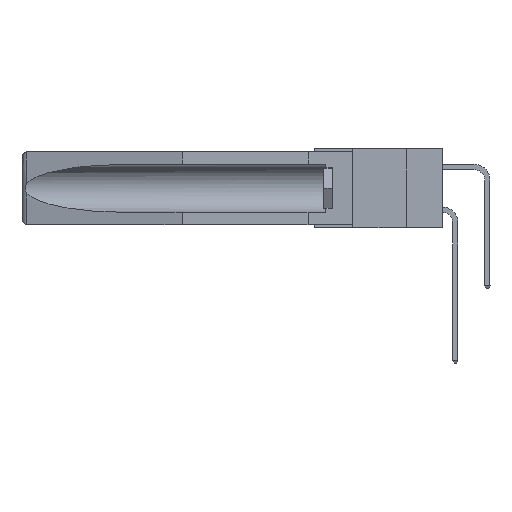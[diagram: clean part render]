
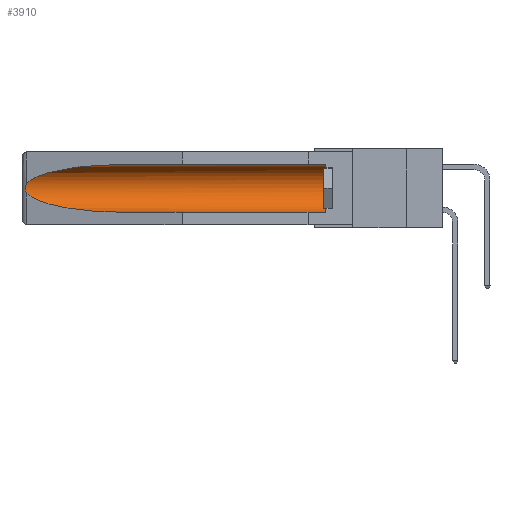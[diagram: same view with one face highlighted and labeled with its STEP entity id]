
A CAD part, left-side view. The second image highlights one B-rep face of the part: STEP entity #3910.
In plain terms, the highlighted cylindrical face has radius 2.857 mm (diameter 5.715 mm), a partial arc.
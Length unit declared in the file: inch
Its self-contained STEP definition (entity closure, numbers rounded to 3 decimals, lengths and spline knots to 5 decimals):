
#23 = CARTESIAN_POINT ( 'NONE',  ( 0.25451, 1.48313, -0.24835 ) ) ;
#266 = ORIENTED_EDGE ( 'NONE', *, *, #12073, .T. ) ;
#439 = EDGE_CURVE ( 'NONE', #23242, #6921, #13004, .T. ) ;
#444 = ORIENTED_EDGE ( 'NONE', *, *, #19345, .F. ) ;
#2038 = DIRECTION ( 'NONE',  ( 0., 0., 1. ) ) ;
#3085 = CARTESIAN_POINT ( 'NONE',  ( 0.26537, 1.52718, -0.14972 ) ) ;
#3279 = DIRECTION ( 'NONE',  ( 0., 1., 0. ) ) ;
#3375 = CARTESIAN_POINT ( 'NONE',  ( 0.26537, 1.52718, -0.19328 ) ) ;
#3388 = LINE ( 'NONE', #18462, #26644 ) ;
#3910 = ADVANCED_FACE ( 'NONE', ( #24500 ), #26945, .F. ) ;
#4541 = CARTESIAN_POINT ( 'NONE',  ( 0.155, 1.07973, -0.284 ) ) ;
#5768 = CARTESIAN_POINT ( 'NONE',  ( 0.155, 1.07973, -0.059 ) ) ;
#5815 = AXIS2_PLACEMENT_3D ( 'NONE', #20556, #8713, #2038 ) ;
#6285 = CIRCLE ( 'NONE', #5815, 0.1125 ) ;
#6734 = CARTESIAN_POINT ( 'NONE',  ( 0.26537, 1.52718, -0.14972 ) ) ;
#6921 = VERTEX_POINT ( 'NONE', #12765 ) ;
#7908 = ORIENTED_EDGE ( 'NONE', *, *, #19481, .T. ) ;
#7948 = VECTOR ( 'NONE', #3279, 39.37008 ) ;
#8572 = EDGE_LOOP ( 'NONE', ( #20658, #13255, #21803, #444, #266, #7908 ) ) ;
#8713 = DIRECTION ( 'NONE',  ( 0., -1., 0. ) ) ;
#8880 = CARTESIAN_POINT ( 'NONE',  ( 0.155, -0.30754, -0.1715 ) ) ;
#9145 = VERTEX_POINT ( 'NONE', #20251 ) ;
#9560 = DIRECTION ( 'NONE',  ( 0., 1., 0. ) ) ;
#9849 = EDGE_CURVE ( 'NONE', #19167, #24347, #11162, .T. ) ;
#10187 = CARTESIAN_POINT ( 'NONE',  ( 0.25451, 1.48313, -0.09465 ) ) ;
#11162 =( BOUNDED_CURVE ( )  B_SPLINE_CURVE ( 3, ( #5768, #23646, #10187, #26009 ),
 .UNSPECIFIED., .F., .F. ) 
 B_SPLINE_CURVE_WITH_KNOTS ( ( 4, 4 ),
 ( 4.71239, 6.08839 ),
 .UNSPECIFIED. ) 
 CURVE ( )  GEOMETRIC_REPRESENTATION_ITEM ( )  RATIONAL_B_SPLINE_CURVE ( ( 1., 0.848, 0.848, 1. ) ) 
 REPRESENTATION_ITEM ( '' )  );
#12073 = EDGE_CURVE ( 'NONE', #9145, #24504, #6285, .T. ) ;
#12416 = CARTESIAN_POINT ( 'NONE',  ( 0.26537, 1.52718, -0.19328 ) ) ;
#12431 = CARTESIAN_POINT ( 'NONE',  ( 0.2675, 1.53308, -0.16763 ) ) ;
#12635 = CARTESIAN_POINT ( 'NONE',  ( 0.26655, 1.53094, -0.18657 ) ) ;
#12765 = CARTESIAN_POINT ( 'NONE',  ( 0.155, 1.07973, -0.284 ) ) ;
#13004 =( BOUNDED_CURVE ( )  B_SPLINE_CURVE ( 3, ( #27343, #23, #18248, #4541 ),
 .UNSPECIFIED., .F., .F. ) 
 B_SPLINE_CURVE_WITH_KNOTS ( ( 4, 4 ),
 ( 0.1948, 1.5708 ),
 .UNSPECIFIED. ) 
 CURVE ( )  GEOMETRIC_REPRESENTATION_ITEM ( )  RATIONAL_B_SPLINE_CURVE ( ( 1., 0.848, 0.848, 1. ) ) 
 REPRESENTATION_ITEM ( '' )  );
#13255 = ORIENTED_EDGE ( 'NONE', *, *, #19354, .T. ) ;
#14329 = B_SPLINE_CURVE_WITH_KNOTS ( 'NONE', 3,
 ( #3085, #16304, #20832, #19144, #12431, #16883, #16688, #12635, #17081, #3375 ),
 .UNSPECIFIED., .F., .F.,
 ( 4, 2, 2, 2, 4 ),
 ( 0., 0.00029, 0.00058, 0.00087, 0.00117 ),
 .UNSPECIFIED. ) ;
#14408 = AXIS2_PLACEMENT_3D ( 'NONE', #8880, #20016, #24511 ) ;
#16304 = CARTESIAN_POINT ( 'NONE',  ( 0.26597, 1.52961, -0.15275 ) ) ;
#16348 = CARTESIAN_POINT ( 'NONE',  ( 0.155, 0.126, -0.059 ) ) ;
#16688 = CARTESIAN_POINT ( 'NONE',  ( 0.2673, 1.53269, -0.17917 ) ) ;
#16793 = LINE ( 'NONE', #25758, #7948 ) ;
#16883 = CARTESIAN_POINT ( 'NONE',  ( 0.2675, 1.53308, -0.17534 ) ) ;
#17081 = CARTESIAN_POINT ( 'NONE',  ( 0.26597, 1.5296, -0.19026 ) ) ;
#18248 = CARTESIAN_POINT ( 'NONE',  ( 0.21114, 1.30732, -0.284 ) ) ;
#18462 = CARTESIAN_POINT ( 'NONE',  ( 0.155, -0.30754, -0.284 ) ) ;
#19144 = CARTESIAN_POINT ( 'NONE',  ( 0.2673, 1.5327, -0.16383 ) ) ;
#19167 = VERTEX_POINT ( 'NONE', #23484 ) ;
#19345 = EDGE_CURVE ( 'NONE', #9145, #6921, #3388, .T. ) ;
#19354 = EDGE_CURVE ( 'NONE', #24347, #23242, #14329, .T. ) ;
#19481 = EDGE_CURVE ( 'NONE', #24504, #19167, #16793, .T. ) ;
#20016 = DIRECTION ( 'NONE',  ( 0., 1., 0. ) ) ;
#20251 = CARTESIAN_POINT ( 'NONE',  ( 0.155, 0.126, -0.284 ) ) ;
#20556 = CARTESIAN_POINT ( 'NONE',  ( 0.155, 0.126, -0.1715 ) ) ;
#20658 = ORIENTED_EDGE ( 'NONE', *, *, #9849, .T. ) ;
#20832 = CARTESIAN_POINT ( 'NONE',  ( 0.26654, 1.53092, -0.15636 ) ) ;
#21803 = ORIENTED_EDGE ( 'NONE', *, *, #439, .T. ) ;
#23242 = VERTEX_POINT ( 'NONE', #12416 ) ;
#23484 = CARTESIAN_POINT ( 'NONE',  ( 0.155, 1.07973, -0.059 ) ) ;
#23646 = CARTESIAN_POINT ( 'NONE',  ( 0.21114, 1.30732, -0.059 ) ) ;
#24347 = VERTEX_POINT ( 'NONE', #6734 ) ;
#24500 = FACE_OUTER_BOUND ( 'NONE', #8572, .T. ) ;
#24504 = VERTEX_POINT ( 'NONE', #16348 ) ;
#24511 = DIRECTION ( 'NONE',  ( 0., 0., 1. ) ) ;
#25758 = CARTESIAN_POINT ( 'NONE',  ( 0.155, -0.30754, -0.059 ) ) ;
#26009 = CARTESIAN_POINT ( 'NONE',  ( 0.26537, 1.52718, -0.14972 ) ) ;
#26644 = VECTOR ( 'NONE', #9560, 39.37008 ) ;
#26945 = CYLINDRICAL_SURFACE ( 'NONE', #14408, 0.1125 ) ;
#27343 = CARTESIAN_POINT ( 'NONE',  ( 0.26537, 1.52718, -0.19328 ) ) ;
